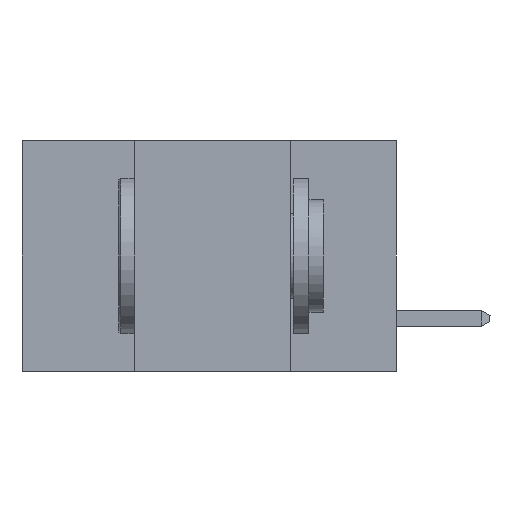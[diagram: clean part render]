
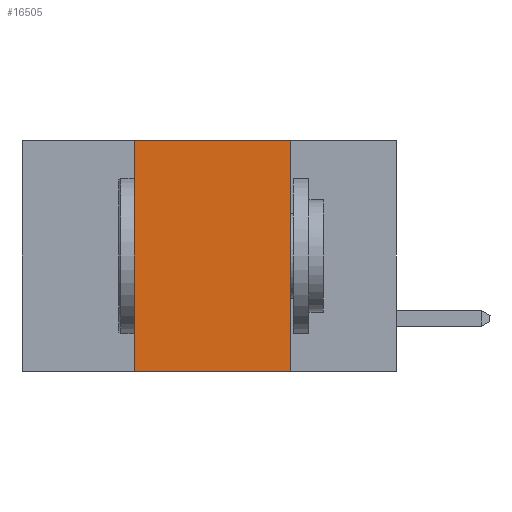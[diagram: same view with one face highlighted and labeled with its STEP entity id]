
A CAD part, left-side view. The second image highlights one B-rep face of the part: STEP entity #16505.
In plain terms, the highlighted planar face has unit normal (-1, 0, 0).
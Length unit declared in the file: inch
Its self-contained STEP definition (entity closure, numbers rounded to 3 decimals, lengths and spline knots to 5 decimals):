
#370 = ORIENTED_EDGE ( 'NONE', *, *, #7926, .F. ) ;
#404 = PLANE ( 'NONE',  #7042 ) ;
#882 = DIRECTION ( 'NONE',  ( 0., -1., 0. ) ) ;
#965 = VECTOR ( 'NONE', #9766, 39.37008 ) ;
#2000 = EDGE_LOOP ( 'NONE', ( #8356, #12632, #370, #13788 ) ) ;
#2258 = DIRECTION ( 'NONE',  ( 0., 0., 1. ) ) ;
#2353 = VECTOR ( 'NONE', #2258, 39.37008 ) ;
#2684 = VECTOR ( 'NONE', #882, 39.37008 ) ;
#4013 = CARTESIAN_POINT ( 'NONE',  ( 0., 0.42, -0.37 ) ) ;
#4288 = VERTEX_POINT ( 'NONE', #13203 ) ;
#5105 = LINE ( 'NONE', #4013, #2353 ) ;
#6783 = LINE ( 'NONE', #18289, #13247 ) ;
#7042 = AXIS2_PLACEMENT_3D ( 'NONE', #13643, #11010, #17064 ) ;
#7926 = EDGE_CURVE ( 'NONE', #14206, #17693, #5105, .T. ) ;
#8279 = CARTESIAN_POINT ( 'NONE',  ( 0., 0.6, 0. ) ) ;
#8290 = EDGE_CURVE ( 'NONE', #17693, #9443, #15779, .T. ) ;
#8309 = CARTESIAN_POINT ( 'NONE',  ( 0., 0.42, -0.37 ) ) ;
#8356 = ORIENTED_EDGE ( 'NONE', *, *, #9999, .F. ) ;
#9443 = VERTEX_POINT ( 'NONE', #17044 ) ;
#9714 = CARTESIAN_POINT ( 'NONE',  ( 0., 0.42, 0. ) ) ;
#9766 = DIRECTION ( 'NONE',  ( 0., -1., 0. ) ) ;
#9999 = EDGE_CURVE ( 'NONE', #9443, #4288, #6783, .T. ) ;
#10051 = LINE ( 'NONE', #18735, #965 ) ;
#11010 = DIRECTION ( 'NONE',  ( 1., 0., 0. ) ) ;
#12632 = ORIENTED_EDGE ( 'NONE', *, *, #8290, .F. ) ;
#12715 = DIRECTION ( 'NONE',  ( 0., 0., -1. ) ) ;
#13203 = CARTESIAN_POINT ( 'NONE',  ( 0., 0.17, -0.37 ) ) ;
#13247 = VECTOR ( 'NONE', #12715, 39.37008 ) ;
#13643 = CARTESIAN_POINT ( 'NONE',  ( 0., 0.6, 0. ) ) ;
#13743 = FACE_OUTER_BOUND ( 'NONE', #2000, .T. ) ;
#13788 = ORIENTED_EDGE ( 'NONE', *, *, #14936, .T. ) ;
#14206 = VERTEX_POINT ( 'NONE', #8309 ) ;
#14936 = EDGE_CURVE ( 'NONE', #14206, #4288, #10051, .T. ) ;
#15779 = LINE ( 'NONE', #8279, #2684 ) ;
#16505 = ADVANCED_FACE ( 'NONE', ( #13743 ), #404, .F. ) ;
#17044 = CARTESIAN_POINT ( 'NONE',  ( 0., 0.17, 0. ) ) ;
#17064 = DIRECTION ( 'NONE',  ( 0., 0., -1. ) ) ;
#17693 = VERTEX_POINT ( 'NONE', #9714 ) ;
#18289 = CARTESIAN_POINT ( 'NONE',  ( 0., 0.17, -0.37 ) ) ;
#18735 = CARTESIAN_POINT ( 'NONE',  ( 0., 0.6, -0.37 ) ) ;
